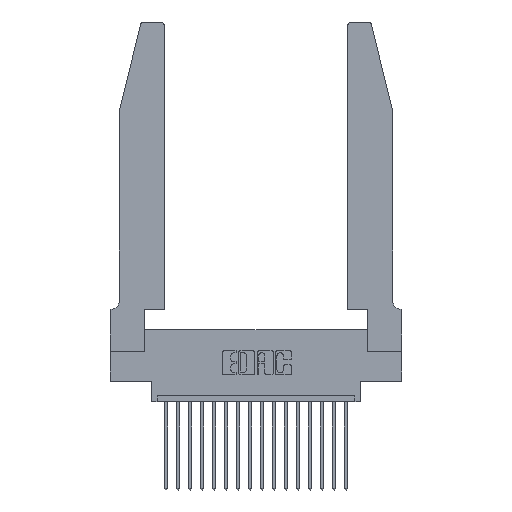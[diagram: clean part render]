
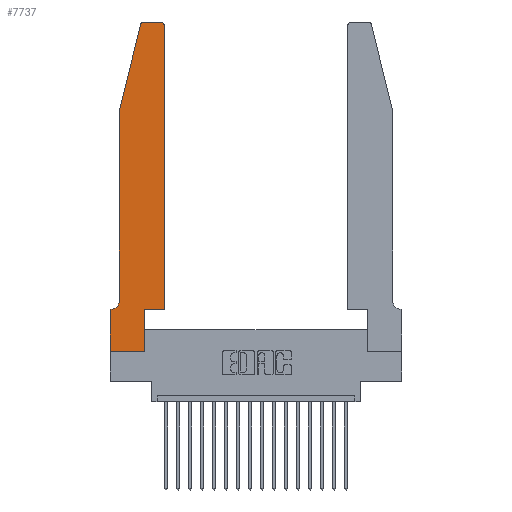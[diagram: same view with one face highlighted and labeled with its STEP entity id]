
A CAD part, top view. The second image highlights one B-rep face of the part: STEP entity #7737.
In plain terms, the highlighted planar face has unit normal (0, 0, 1).
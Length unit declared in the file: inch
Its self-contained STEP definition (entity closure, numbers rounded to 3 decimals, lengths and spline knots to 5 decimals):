
#97 = LINE ( 'NONE', #995, #13174 ) ;
#112 = CARTESIAN_POINT ( 'NONE',  ( 0.2865, 0., 0.37 ) ) ;
#256 = EDGE_CURVE ( 'NONE', #15034, #4475, #3829, .T. ) ;
#286 = CARTESIAN_POINT ( 'NONE',  ( 0., 0., 0.37 ) ) ;
#593 = LINE ( 'NONE', #12745, #1096 ) ;
#758 = DIRECTION ( 'NONE',  ( 0., 1., 0. ) ) ;
#763 = EDGE_CURVE ( 'NONE', #4687, #10543, #19595, .T. ) ;
#857 = VECTOR ( 'NONE', #11814, 39.37008 ) ;
#995 = CARTESIAN_POINT ( 'NONE',  ( 0.2605, 2.75, 0.37 ) ) ;
#1096 = VECTOR ( 'NONE', #14348, 39.37008 ) ;
#1200 = ORIENTED_EDGE ( 'NONE', *, *, #15214, .T. ) ;
#1213 = ORIENTED_EDGE ( 'NONE', *, *, #256, .T. ) ;
#1224 = DIRECTION ( 'NONE',  ( 0., 0., 1. ) ) ;
#1549 = DIRECTION ( 'NONE',  ( 0., 0., -1. ) ) ;
#1802 = DIRECTION ( 'NONE',  ( -0.239, -0.971, 0. ) ) ;
#2227 = ORIENTED_EDGE ( 'NONE', *, *, #9082, .T. ) ;
#2461 = DIRECTION ( 'NONE',  ( 0., -1., 0. ) ) ;
#2963 = CARTESIAN_POINT ( 'NONE',  ( 0.4505, 0.35, 0.37 ) ) ;
#3090 = LINE ( 'NONE', #16787, #20139 ) ;
#3112 = CARTESIAN_POINT ( 'NONE',  ( 0.284, 2.75, 0.37 ) ) ;
#3484 = CARTESIAN_POINT ( 'NONE',  ( 0.0755, 2., 0.37 ) ) ;
#3563 = EDGE_CURVE ( 'NONE', #9767, #20380, #7928, .T. ) ;
#3576 = DIRECTION ( 'NONE',  ( 0., 0., 1. ) ) ;
#3821 = EDGE_CURVE ( 'NONE', #18661, #9230, #97, .T. ) ;
#3829 = LINE ( 'NONE', #18126, #5550 ) ;
#3964 = CIRCLE ( 'NONE', #9538, 0.03 ) ;
#4304 = DIRECTION ( 'NONE',  ( 1., 0., 0. ) ) ;
#4332 = CARTESIAN_POINT ( 'NONE',  ( 0., 0., 0.37 ) ) ;
#4475 = VERTEX_POINT ( 'NONE', #19516 ) ;
#4602 = CARTESIAN_POINT ( 'NONE',  ( 0.0055, 0.42, 0.37 ) ) ;
#4687 = VERTEX_POINT ( 'NONE', #112 ) ;
#5361 = CIRCLE ( 'NONE', #11461, 0.03 ) ;
#5498 = VERTEX_POINT ( 'NONE', #10952 ) ;
#5550 = VECTOR ( 'NONE', #758, 39.37008 ) ;
#5863 = LINE ( 'NONE', #7967, #12741 ) ;
#5938 = PLANE ( 'NONE',  #17221 ) ;
#6126 = EDGE_LOOP ( 'NONE', ( #7240, #10744, #15677, #2227, #12457, #10429, #16103, #7775, #20382, #15290, #1213, #1200 ) ) ;
#6407 = AXIS2_PLACEMENT_3D ( 'NONE', #4602, #1549, #20206 ) ;
#6567 = CARTESIAN_POINT ( 'NONE',  ( 0.2865, 0.35, 0.37 ) ) ;
#6578 = VERTEX_POINT ( 'NONE', #12439 ) ;
#6628 = LINE ( 'NONE', #6813, #13523 ) ;
#6813 = CARTESIAN_POINT ( 'NONE',  ( 0.0755, 0.35, 0.37 ) ) ;
#7160 = EDGE_CURVE ( 'NONE', #10543, #15034, #5863, .T. ) ;
#7240 = ORIENTED_EDGE ( 'NONE', *, *, #3821, .T. ) ;
#7539 = EDGE_CURVE ( 'NONE', #11005, #5498, #7822, .T. ) ;
#7737 = ADVANCED_FACE ( 'NONE', ( #19634 ), #5938, .T. ) ;
#7775 = ORIENTED_EDGE ( 'NONE', *, *, #7855, .T. ) ;
#7798 = CARTESIAN_POINT ( 'NONE',  ( 0.25487, 2.72718, 0.37 ) ) ;
#7822 = LINE ( 'NONE', #3484, #10522 ) ;
#7855 = EDGE_CURVE ( 'NONE', #20380, #4687, #3090, .T. ) ;
#7928 = LINE ( 'NONE', #4332, #15332 ) ;
#7967 = CARTESIAN_POINT ( 'NONE',  ( 0.4505, 0.35, 0.37 ) ) ;
#9082 = EDGE_CURVE ( 'NONE', #5498, #6578, #593, .T. ) ;
#9131 = CARTESIAN_POINT ( 'NONE',  ( 0.0055, 0.35, 0.37 ) ) ;
#9230 = VERTEX_POINT ( 'NONE', #3112 ) ;
#9538 = AXIS2_PLACEMENT_3D ( 'NONE', #15253, #1224, #13864 ) ;
#9767 = VERTEX_POINT ( 'NONE', #15761 ) ;
#9897 = EDGE_CURVE ( 'NONE', #6578, #11307, #11422, .T. ) ;
#10429 = ORIENTED_EDGE ( 'NONE', *, *, #15992, .T. ) ;
#10522 = VECTOR ( 'NONE', #1802, 39.37008 ) ;
#10543 = VERTEX_POINT ( 'NONE', #6567 ) ;
#10744 = ORIENTED_EDGE ( 'NONE', *, *, #18774, .T. ) ;
#10952 = CARTESIAN_POINT ( 'NONE',  ( 0.0755, 2., 0.37 ) ) ;
#11005 = VERTEX_POINT ( 'NONE', #7798 ) ;
#11307 = VERTEX_POINT ( 'NONE', #9131 ) ;
#11422 = CIRCLE ( 'NONE', #6407, 0.07 ) ;
#11461 = AXIS2_PLACEMENT_3D ( 'NONE', #19631, #3576, #17889 ) ;
#11814 = DIRECTION ( 'NONE',  ( 0., 1., 0. ) ) ;
#11958 = CARTESIAN_POINT ( 'NONE',  ( 0.2865, 0.35, 0.37 ) ) ;
#12439 = CARTESIAN_POINT ( 'NONE',  ( 0.0755, 0.42, 0.37 ) ) ;
#12457 = ORIENTED_EDGE ( 'NONE', *, *, #9897, .T. ) ;
#12741 = VECTOR ( 'NONE', #13877, 39.37008 ) ;
#12745 = CARTESIAN_POINT ( 'NONE',  ( 0.0755, 2., 0.37 ) ) ;
#13174 = VECTOR ( 'NONE', #14574, 39.37008 ) ;
#13408 = DIRECTION ( 'NONE',  ( 0., 0., 1. ) ) ;
#13523 = VECTOR ( 'NONE', #16074, 39.37008 ) ;
#13864 = DIRECTION ( 'NONE',  ( 1., 0., 0. ) ) ;
#13877 = DIRECTION ( 'NONE',  ( 1., 0., 0. ) ) ;
#14348 = DIRECTION ( 'NONE',  ( 0., -1., 0. ) ) ;
#14574 = DIRECTION ( 'NONE',  ( -1., 0., 0. ) ) ;
#14895 = CARTESIAN_POINT ( 'NONE',  ( 0.4205, 2.75, 0.37 ) ) ;
#15034 = VERTEX_POINT ( 'NONE', #2963 ) ;
#15214 = EDGE_CURVE ( 'NONE', #4475, #18661, #5361, .T. ) ;
#15253 = CARTESIAN_POINT ( 'NONE',  ( 0.284, 2.72, 0.37 ) ) ;
#15290 = ORIENTED_EDGE ( 'NONE', *, *, #7160, .T. ) ;
#15332 = VECTOR ( 'NONE', #2461, 39.37008 ) ;
#15677 = ORIENTED_EDGE ( 'NONE', *, *, #7539, .T. ) ;
#15761 = CARTESIAN_POINT ( 'NONE',  ( 0., 0.35, 0.37 ) ) ;
#15992 = EDGE_CURVE ( 'NONE', #11307, #9767, #6628, .T. ) ;
#16074 = DIRECTION ( 'NONE',  ( -1., 0., 0. ) ) ;
#16089 = CARTESIAN_POINT ( 'NONE',  ( 0., 0.35, 0.37 ) ) ;
#16103 = ORIENTED_EDGE ( 'NONE', *, *, #3563, .T. ) ;
#16787 = CARTESIAN_POINT ( 'NONE',  ( 0., 0., 0.37 ) ) ;
#17221 = AXIS2_PLACEMENT_3D ( 'NONE', #16089, #13408, #4304 ) ;
#17889 = DIRECTION ( 'NONE',  ( 1., 0., 0. ) ) ;
#18126 = CARTESIAN_POINT ( 'NONE',  ( 0.4505, 0.35, 0.37 ) ) ;
#18661 = VERTEX_POINT ( 'NONE', #14895 ) ;
#18774 = EDGE_CURVE ( 'NONE', #9230, #11005, #3964, .T. ) ;
#19516 = CARTESIAN_POINT ( 'NONE',  ( 0.4505, 2.72, 0.37 ) ) ;
#19595 = LINE ( 'NONE', #11958, #857 ) ;
#19631 = CARTESIAN_POINT ( 'NONE',  ( 0.4205, 2.72, 0.37 ) ) ;
#19634 = FACE_OUTER_BOUND ( 'NONE', #6126, .T. ) ;
#19952 = DIRECTION ( 'NONE',  ( 1., 0., 0. ) ) ;
#20139 = VECTOR ( 'NONE', #19952, 39.37008 ) ;
#20206 = DIRECTION ( 'NONE',  ( -1., 0., 0. ) ) ;
#20380 = VERTEX_POINT ( 'NONE', #286 ) ;
#20382 = ORIENTED_EDGE ( 'NONE', *, *, #763, .T. ) ;
